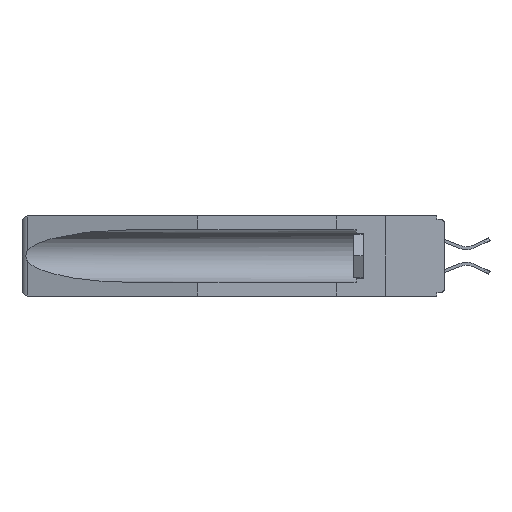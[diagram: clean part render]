
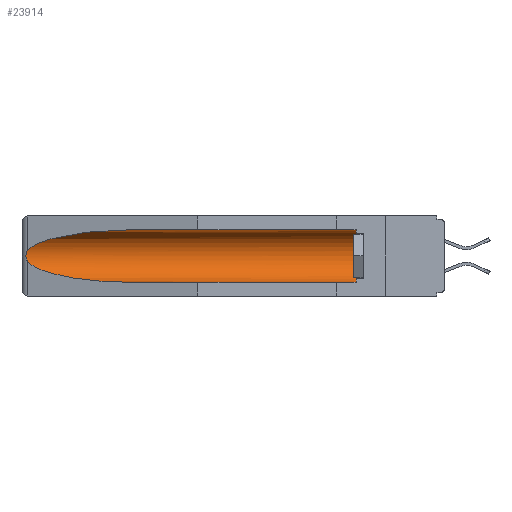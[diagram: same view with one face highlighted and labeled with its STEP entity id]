
A CAD part, left-side view. The second image highlights one B-rep face of the part: STEP entity #23914.
In plain terms, the highlighted cylindrical face has radius 2.857 mm (diameter 5.715 mm), a partial arc.
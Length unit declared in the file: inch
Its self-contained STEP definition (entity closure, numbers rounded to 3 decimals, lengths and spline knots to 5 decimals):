
#414 = CARTESIAN_POINT ( 'NONE',  ( 0.26537, 1.52718, -0.14972 ) ) ;
#867 = CARTESIAN_POINT ( 'NONE',  ( 0.21114, 1.30732, -0.059 ) ) ;
#1161 = CARTESIAN_POINT ( 'NONE',  ( 0.155, -0.30754, -0.1715 ) ) ;
#1712 = EDGE_CURVE ( 'NONE', #13414, #11100, #17764, .T. ) ;
#2541 = CARTESIAN_POINT ( 'NONE',  ( 0.26597, 1.5296, -0.19026 ) ) ;
#2801 = DIRECTION ( 'NONE',  ( 0., 1., 0. ) ) ;
#3631 = EDGE_CURVE ( 'NONE', #11100, #8217, #13567, .T. ) ;
#3653 = ORIENTED_EDGE ( 'NONE', *, *, #19541, .T. ) ;
#4460 = AXIS2_PLACEMENT_3D ( 'NONE', #1161, #2801, #12486 ) ;
#4886 = CARTESIAN_POINT ( 'NONE',  ( 0.21114, 1.30732, -0.284 ) ) ;
#5485 = DIRECTION ( 'NONE',  ( 0., 0., 1. ) ) ;
#5635 = ORIENTED_EDGE ( 'NONE', *, *, #10991, .F. ) ;
#5897 = VECTOR ( 'NONE', #6531, 39.37008 ) ;
#6073 = CARTESIAN_POINT ( 'NONE',  ( 0.2675, 1.53308, -0.16763 ) ) ;
#6376 = VERTEX_POINT ( 'NONE', #23353 ) ;
#6384 = CYLINDRICAL_SURFACE ( 'NONE', #4460, 0.1125 ) ;
#6531 = DIRECTION ( 'NONE',  ( 0., 1., 0. ) ) ;
#6935 = CARTESIAN_POINT ( 'NONE',  ( 0.26537, 1.52718, -0.14972 ) ) ;
#7682 = B_SPLINE_CURVE_WITH_KNOTS ( 'NONE', 3,
 ( #414, #19511, #17620, #21729, #6073, #19774, #10208, #8170, #2541, #19591 ),
 .UNSPECIFIED., .F., .F.,
 ( 4, 2, 2, 2, 4 ),
 ( 0., 0.00029, 0.00058, 0.00087, 0.00117 ),
 .UNSPECIFIED. ) ;
#8170 = CARTESIAN_POINT ( 'NONE',  ( 0.26655, 1.53094, -0.18657 ) ) ;
#8217 = VERTEX_POINT ( 'NONE', #15188 ) ;
#8686 = EDGE_LOOP ( 'NONE', ( #9994, #11308, #24803, #5635, #3653, #19181 ) ) ;
#9678 = CARTESIAN_POINT ( 'NONE',  ( 0.155, 0.126, -0.059 ) ) ;
#9843 = DIRECTION ( 'NONE',  ( 0., 1., 0. ) ) ;
#9994 = ORIENTED_EDGE ( 'NONE', *, *, #3631, .T. ) ;
#10169 = VERTEX_POINT ( 'NONE', #15666 ) ;
#10208 = CARTESIAN_POINT ( 'NONE',  ( 0.2673, 1.53269, -0.17917 ) ) ;
#10715 = CARTESIAN_POINT ( 'NONE',  ( 0.25451, 1.48313, -0.24835 ) ) ;
#10991 = EDGE_CURVE ( 'NONE', #6376, #10169, #16162, .T. ) ;
#11100 = VERTEX_POINT ( 'NONE', #13272 ) ;
#11308 = ORIENTED_EDGE ( 'NONE', *, *, #20444, .T. ) ;
#11406 = CARTESIAN_POINT ( 'NONE',  ( 0.155, 0.126, -0.1715 ) ) ;
#12486 = DIRECTION ( 'NONE',  ( 0., 0., 1. ) ) ;
#13244 = CIRCLE ( 'NONE', #18964, 0.1125 ) ;
#13272 = CARTESIAN_POINT ( 'NONE',  ( 0.155, 1.07973, -0.059 ) ) ;
#13414 = VERTEX_POINT ( 'NONE', #9678 ) ;
#13567 =( BOUNDED_CURVE ( )  B_SPLINE_CURVE ( 3, ( #24140, #867, #14612, #6935 ),
 .UNSPECIFIED., .F., .F. ) 
 B_SPLINE_CURVE_WITH_KNOTS ( ( 4, 4 ),
 ( 4.71239, 6.08839 ),
 .UNSPECIFIED. ) 
 CURVE ( )  GEOMETRIC_REPRESENTATION_ITEM ( )  RATIONAL_B_SPLINE_CURVE ( ( 1., 0.848, 0.848, 1. ) ) 
 REPRESENTATION_ITEM ( '' )  );
#14612 = CARTESIAN_POINT ( 'NONE',  ( 0.25451, 1.48313, -0.09465 ) ) ;
#15188 = CARTESIAN_POINT ( 'NONE',  ( 0.26537, 1.52718, -0.14972 ) ) ;
#15341 = VECTOR ( 'NONE', #9843, 39.37008 ) ;
#15666 = CARTESIAN_POINT ( 'NONE',  ( 0.155, 1.07973, -0.284 ) ) ;
#16143 = CARTESIAN_POINT ( 'NONE',  ( 0.155, -0.30754, -0.284 ) ) ;
#16162 = LINE ( 'NONE', #16143, #5897 ) ;
#17620 = CARTESIAN_POINT ( 'NONE',  ( 0.26654, 1.53092, -0.15636 ) ) ;
#17764 = LINE ( 'NONE', #21453, #15341 ) ;
#18399 = CARTESIAN_POINT ( 'NONE',  ( 0.155, 1.07973, -0.284 ) ) ;
#18964 = AXIS2_PLACEMENT_3D ( 'NONE', #11406, #20981, #5485 ) ;
#19035 = CARTESIAN_POINT ( 'NONE',  ( 0.26537, 1.52718, -0.19328 ) ) ;
#19181 = ORIENTED_EDGE ( 'NONE', *, *, #1712, .T. ) ;
#19316 =( BOUNDED_CURVE ( )  B_SPLINE_CURVE ( 3, ( #20280, #10715, #4886, #18399 ),
 .UNSPECIFIED., .F., .F. ) 
 B_SPLINE_CURVE_WITH_KNOTS ( ( 4, 4 ),
 ( 0.1948, 1.5708 ),
 .UNSPECIFIED. ) 
 CURVE ( )  GEOMETRIC_REPRESENTATION_ITEM ( )  RATIONAL_B_SPLINE_CURVE ( ( 1., 0.848, 0.848, 1. ) ) 
 REPRESENTATION_ITEM ( '' )  );
#19511 = CARTESIAN_POINT ( 'NONE',  ( 0.26597, 1.52961, -0.15275 ) ) ;
#19541 = EDGE_CURVE ( 'NONE', #6376, #13414, #13244, .T. ) ;
#19591 = CARTESIAN_POINT ( 'NONE',  ( 0.26537, 1.52718, -0.19328 ) ) ;
#19774 = CARTESIAN_POINT ( 'NONE',  ( 0.2675, 1.53308, -0.17534 ) ) ;
#20280 = CARTESIAN_POINT ( 'NONE',  ( 0.26537, 1.52718, -0.19328 ) ) ;
#20444 = EDGE_CURVE ( 'NONE', #8217, #24038, #7682, .T. ) ;
#20981 = DIRECTION ( 'NONE',  ( 0., -1., 0. ) ) ;
#21453 = CARTESIAN_POINT ( 'NONE',  ( 0.155, -0.30754, -0.059 ) ) ;
#21729 = CARTESIAN_POINT ( 'NONE',  ( 0.2673, 1.5327, -0.16383 ) ) ;
#22587 = EDGE_CURVE ( 'NONE', #24038, #10169, #19316, .T. ) ;
#23353 = CARTESIAN_POINT ( 'NONE',  ( 0.155, 0.126, -0.284 ) ) ;
#23667 = FACE_OUTER_BOUND ( 'NONE', #8686, .T. ) ;
#23914 = ADVANCED_FACE ( 'NONE', ( #23667 ), #6384, .F. ) ;
#24038 = VERTEX_POINT ( 'NONE', #19035 ) ;
#24140 = CARTESIAN_POINT ( 'NONE',  ( 0.155, 1.07973, -0.059 ) ) ;
#24803 = ORIENTED_EDGE ( 'NONE', *, *, #22587, .T. ) ;
